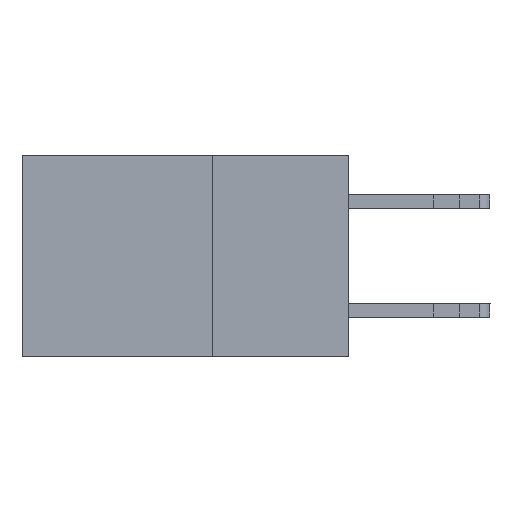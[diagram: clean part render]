
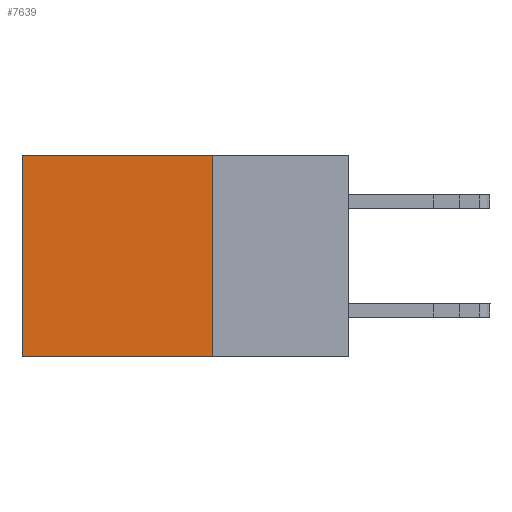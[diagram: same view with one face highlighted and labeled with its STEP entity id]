
A CAD part, left-side view. The second image highlights one B-rep face of the part: STEP entity #7639.
In plain terms, the highlighted planar face has unit normal (-1, 0, 0).
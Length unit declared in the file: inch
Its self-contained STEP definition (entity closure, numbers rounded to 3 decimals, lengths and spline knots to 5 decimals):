
#403 = PLANE ( 'NONE',  #6958 ) ;
#505 = FACE_OUTER_BOUND ( 'NONE', #1604, .T. ) ;
#721 = DIRECTION ( 'NONE',  ( 0., 0., -1. ) ) ;
#1293 = CARTESIAN_POINT ( 'NONE',  ( 0.2615, 0.6, -0.37 ) ) ;
#1357 = VERTEX_POINT ( 'NONE', #2385 ) ;
#1604 = EDGE_LOOP ( 'NONE', ( #3268, #3324, #9853, #10819 ) ) ;
#1617 = DIRECTION ( 'NONE',  ( 0., 0., -1. ) ) ;
#1746 = LINE ( 'NONE', #3239, #7363 ) ;
#1840 = EDGE_CURVE ( 'NONE', #10815, #1357, #10677, .T. ) ;
#1930 = DIRECTION ( 'NONE',  ( 0., 1., 0. ) ) ;
#2141 = VECTOR ( 'NONE', #721, 39.37008 ) ;
#2385 = CARTESIAN_POINT ( 'NONE',  ( 0.2615, 0.6, 0. ) ) ;
#2489 = CARTESIAN_POINT ( 'NONE',  ( 0.2615, 0.25, 0. ) ) ;
#3239 = CARTESIAN_POINT ( 'NONE',  ( 0.2615, 0.25, -0.37 ) ) ;
#3268 = ORIENTED_EDGE ( 'NONE', *, *, #10355, .T. ) ;
#3324 = ORIENTED_EDGE ( 'NONE', *, *, #10509, .F. ) ;
#3598 = VECTOR ( 'NONE', #6301, 39.37008 ) ;
#4865 = CARTESIAN_POINT ( 'NONE',  ( 0.2615, 0.25, 0. ) ) ;
#4977 = VERTEX_POINT ( 'NONE', #1293 ) ;
#4992 = VECTOR ( 'NONE', #1930, 39.37008 ) ;
#6301 = DIRECTION ( 'NONE',  ( 0., 0., -1. ) ) ;
#6958 = AXIS2_PLACEMENT_3D ( 'NONE', #9270, #8267, #1617 ) ;
#7363 = VECTOR ( 'NONE', #9702, 39.37008 ) ;
#7639 = ADVANCED_FACE ( 'NONE', ( #505 ), #403, .F. ) ;
#8267 = DIRECTION ( 'NONE',  ( 1., 0., 0. ) ) ;
#8374 = VERTEX_POINT ( 'NONE', #9391 ) ;
#8514 = CARTESIAN_POINT ( 'NONE',  ( 0.2615, 0.25, -0.37 ) ) ;
#9121 = EDGE_CURVE ( 'NONE', #10815, #8374, #10552, .T. ) ;
#9270 = CARTESIAN_POINT ( 'NONE',  ( 0.2615, 0.25, -0.37 ) ) ;
#9391 = CARTESIAN_POINT ( 'NONE',  ( 0.2615, 0.25, -0.37 ) ) ;
#9472 = CARTESIAN_POINT ( 'NONE',  ( 0.2615, 0.6, -0.37 ) ) ;
#9702 = DIRECTION ( 'NONE',  ( 0., 1., 0. ) ) ;
#9853 = ORIENTED_EDGE ( 'NONE', *, *, #9121, .F. ) ;
#10355 = EDGE_CURVE ( 'NONE', #1357, #4977, #11837, .T. ) ;
#10509 = EDGE_CURVE ( 'NONE', #8374, #4977, #1746, .T. ) ;
#10552 = LINE ( 'NONE', #8514, #2141 ) ;
#10677 = LINE ( 'NONE', #2489, #4992 ) ;
#10815 = VERTEX_POINT ( 'NONE', #4865 ) ;
#10819 = ORIENTED_EDGE ( 'NONE', *, *, #1840, .T. ) ;
#11837 = LINE ( 'NONE', #9472, #3598 ) ;
